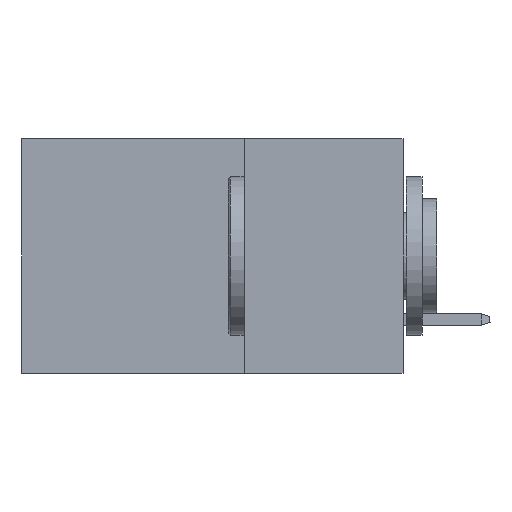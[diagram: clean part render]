
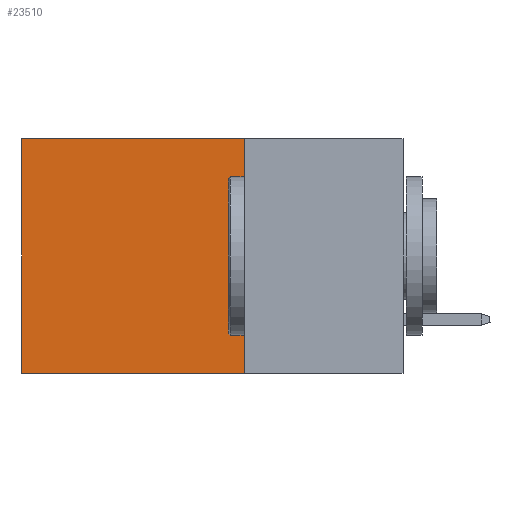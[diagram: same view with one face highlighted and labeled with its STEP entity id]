
A CAD part, left-side view. The second image highlights one B-rep face of the part: STEP entity #23510.
In plain terms, the highlighted planar face has unit normal (-1, 0, 0).
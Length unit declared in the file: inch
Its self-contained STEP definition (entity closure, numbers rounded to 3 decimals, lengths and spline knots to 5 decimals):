
#390 = ORIENTED_EDGE ( 'NONE', *, *, #7388, .T. ) ;
#3920 = LINE ( 'NONE', #46911, #30379 ) ;
#7388 = EDGE_CURVE ( 'NONE', #11427, #17330, #3920, .T. ) ;
#7622 = CARTESIAN_POINT ( 'NONE',  ( 0.2875, 0.6, 0. ) ) ;
#7710 = CARTESIAN_POINT ( 'NONE',  ( 0.2875, 0.25, -0.37 ) ) ;
#8065 = DIRECTION ( 'NONE',  ( 1., 0., 0. ) ) ;
#8297 = CARTESIAN_POINT ( 'NONE',  ( 0.2875, 0.25, 0. ) ) ;
#8373 = VERTEX_POINT ( 'NONE', #44380 ) ;
#8784 = LINE ( 'NONE', #27179, #28790 ) ;
#10341 = CARTESIAN_POINT ( 'NONE',  ( 0.2875, 0.25, 0. ) ) ;
#11427 = VERTEX_POINT ( 'NONE', #10341 ) ;
#11534 = ORIENTED_EDGE ( 'NONE', *, *, #15395, .T. ) ;
#11883 = FACE_OUTER_BOUND ( 'NONE', #16614, .T. ) ;
#13192 = AXIS2_PLACEMENT_3D ( 'NONE', #8297, #8065, #19532 ) ;
#13761 = DIRECTION ( 'NONE',  ( 0., 1., 0. ) ) ;
#15101 = VERTEX_POINT ( 'NONE', #37688 ) ;
#15357 = LINE ( 'NONE', #7710, #40480 ) ;
#15395 = EDGE_CURVE ( 'NONE', #17330, #15101, #26020, .T. ) ;
#16614 = EDGE_LOOP ( 'NONE', ( #11534, #35730, #29247, #390 ) ) ;
#17330 = VERTEX_POINT ( 'NONE', #33834 ) ;
#19532 = DIRECTION ( 'NONE',  ( 0., 0., -1. ) ) ;
#19591 = EDGE_CURVE ( 'NONE', #8373, #15101, #15357, .T. ) ;
#23510 = ADVANCED_FACE ( 'NONE', ( #11883 ), #26453, .F. ) ;
#26020 = LINE ( 'NONE', #7622, #44663 ) ;
#26453 = PLANE ( 'NONE',  #13192 ) ;
#27179 = CARTESIAN_POINT ( 'NONE',  ( 0.2875, 0.25, 0. ) ) ;
#28490 = EDGE_CURVE ( 'NONE', #11427, #8373, #8784, .T. ) ;
#28790 = VECTOR ( 'NONE', #37905, 39.37008 ) ;
#29247 = ORIENTED_EDGE ( 'NONE', *, *, #28490, .F. ) ;
#30379 = VECTOR ( 'NONE', #39747, 39.37008 ) ;
#33834 = CARTESIAN_POINT ( 'NONE',  ( 0.2875, 0.6, 0. ) ) ;
#35730 = ORIENTED_EDGE ( 'NONE', *, *, #19591, .F. ) ;
#37688 = CARTESIAN_POINT ( 'NONE',  ( 0.2875, 0.6, -0.37 ) ) ;
#37905 = DIRECTION ( 'NONE',  ( 0., 0., -1. ) ) ;
#39747 = DIRECTION ( 'NONE',  ( 0., 1., 0. ) ) ;
#40480 = VECTOR ( 'NONE', #13761, 39.37008 ) ;
#40559 = DIRECTION ( 'NONE',  ( 0., 0., -1. ) ) ;
#44380 = CARTESIAN_POINT ( 'NONE',  ( 0.2875, 0.25, -0.37 ) ) ;
#44663 = VECTOR ( 'NONE', #40559, 39.37008 ) ;
#46911 = CARTESIAN_POINT ( 'NONE',  ( 0.2875, 0.25, 0. ) ) ;
